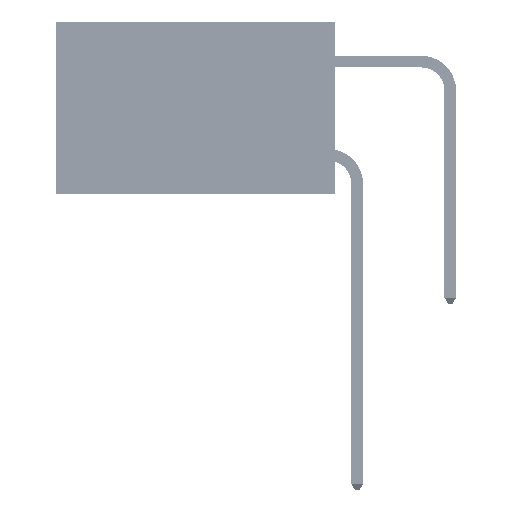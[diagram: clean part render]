
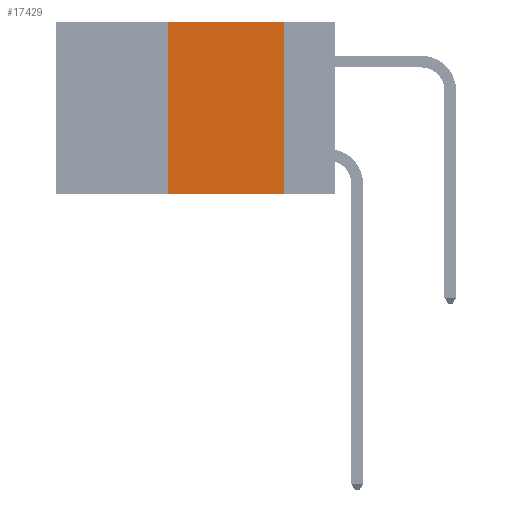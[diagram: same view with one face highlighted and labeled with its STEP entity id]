
A CAD part, left-side view. The second image highlights one B-rep face of the part: STEP entity #17429.
In plain terms, the highlighted planar face has unit normal (-1, 0, 0).
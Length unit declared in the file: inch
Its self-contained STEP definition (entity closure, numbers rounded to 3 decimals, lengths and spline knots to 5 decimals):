
#1898 = DIRECTION ( 'NONE',  ( 0., 0., -1. ) ) ;
#2973 = VECTOR ( 'NONE', #19436, 39.37008 ) ;
#3287 = DIRECTION ( 'NONE',  ( 0., 0., 1. ) ) ;
#3533 = DIRECTION ( 'NONE',  ( 0., 0., -1. ) ) ;
#3606 = CARTESIAN_POINT ( 'NONE',  ( 0., 0.36, 0. ) ) ;
#4242 = VERTEX_POINT ( 'NONE', #27590 ) ;
#4377 = VECTOR ( 'NONE', #10750, 39.37008 ) ;
#4938 = VERTEX_POINT ( 'NONE', #29606 ) ;
#6796 = VERTEX_POINT ( 'NONE', #23626 ) ;
#7296 = PLANE ( 'NONE',  #8968 ) ;
#8968 = AXIS2_PLACEMENT_3D ( 'NONE', #25791, #44389, #3533 ) ;
#9049 = LINE ( 'NONE', #25637, #4377 ) ;
#9334 = EDGE_CURVE ( 'NONE', #4938, #4242, #33398, .T. ) ;
#10750 = DIRECTION ( 'NONE',  ( 0., -1., 0. ) ) ;
#11770 = LINE ( 'NONE', #11907, #2973 ) ;
#11907 = CARTESIAN_POINT ( 'NONE',  ( 0., 0.6, 0. ) ) ;
#13489 = VECTOR ( 'NONE', #3287, 39.37008 ) ;
#17215 = EDGE_CURVE ( 'NONE', #38384, #6796, #35029, .T. ) ;
#17429 = ADVANCED_FACE ( 'NONE', ( #27014 ), #7296, .F. ) ;
#19255 = ORIENTED_EDGE ( 'NONE', *, *, #27657, .T. ) ;
#19436 = DIRECTION ( 'NONE',  ( 0., -1., 0. ) ) ;
#19468 = EDGE_CURVE ( 'NONE', #4242, #38384, #11770, .T. ) ;
#20874 = ORIENTED_EDGE ( 'NONE', *, *, #9334, .F. ) ;
#23626 = CARTESIAN_POINT ( 'NONE',  ( 0., 0.11, -0.37 ) ) ;
#24319 = CARTESIAN_POINT ( 'NONE',  ( 0., 0.11, 0. ) ) ;
#25637 = CARTESIAN_POINT ( 'NONE',  ( 0., 0.6, -0.37 ) ) ;
#25791 = CARTESIAN_POINT ( 'NONE',  ( 0., 0.6, 0. ) ) ;
#27014 = FACE_OUTER_BOUND ( 'NONE', #47416, .T. ) ;
#27590 = CARTESIAN_POINT ( 'NONE',  ( 0., 0.36, 0. ) ) ;
#27657 = EDGE_CURVE ( 'NONE', #4938, #6796, #9049, .T. ) ;
#29606 = CARTESIAN_POINT ( 'NONE',  ( 0., 0.36, -0.37 ) ) ;
#33398 = LINE ( 'NONE', #3606, #13489 ) ;
#35029 = LINE ( 'NONE', #24319, #43235 ) ;
#38384 = VERTEX_POINT ( 'NONE', #43991 ) ;
#40524 = ORIENTED_EDGE ( 'NONE', *, *, #17215, .F. ) ;
#43235 = VECTOR ( 'NONE', #1898, 39.37008 ) ;
#43991 = CARTESIAN_POINT ( 'NONE',  ( 0., 0.11, 0. ) ) ;
#44389 = DIRECTION ( 'NONE',  ( 1., 0., 0. ) ) ;
#44510 = ORIENTED_EDGE ( 'NONE', *, *, #19468, .F. ) ;
#47416 = EDGE_LOOP ( 'NONE', ( #40524, #44510, #20874, #19255 ) ) ;
